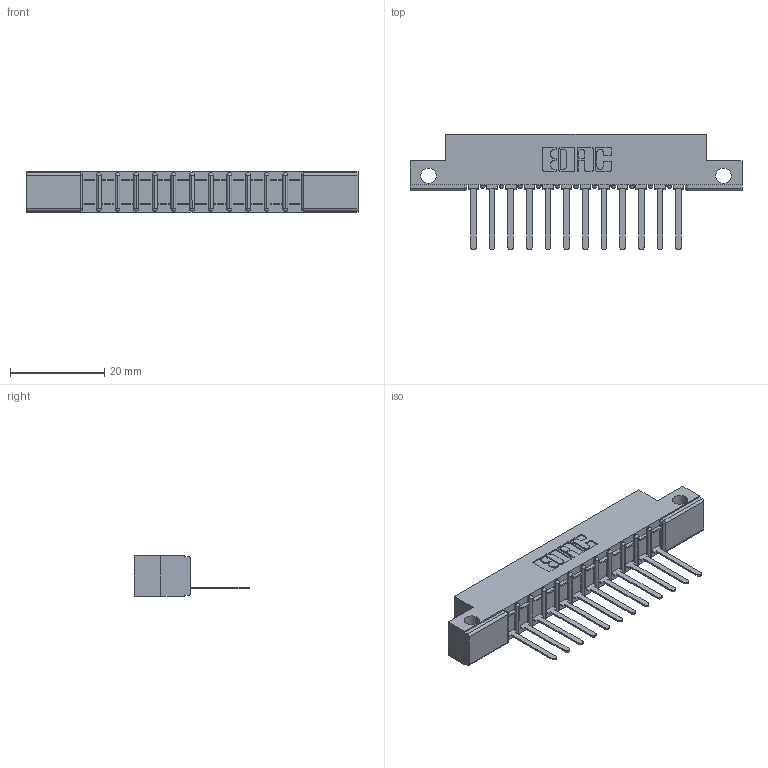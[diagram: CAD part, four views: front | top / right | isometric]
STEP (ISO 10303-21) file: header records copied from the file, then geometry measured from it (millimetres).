
FILE_DESCRIPTION (( 'STEP AP203' ), '1' );
FILE_NAME ('357-012-541-112.STEP', '2019-09-16T19:13:20', ( '' ), ( '' ), 'SwSTEP 2.0', 'SolidWorks 2016', '' );
FILE_SCHEMA (( 'CONFIG_CONTROL_DESIGN' ));
Length unit declared in the file: inch
Products named in the file (3): 307 Part_.128 Dia Side Mounting Holes; 307-290-002_541; 357-012-541-112
Assembly tree (13 placements, depth 2):
  357-012-541-112
    307 Part_.128 Dia Side Mounting Holes
    307-290-002_541  x12
Bounding box: 70.56 x 24.59 x 8.71 mm (x, y, z)
Volume: 4611 mm3; surface area: 7897.6 mm2
Topology: 13 solids, 13 shells, 1019 faces, 3107 edges, 2034 vertices
Faces by surface type: plane 610, cylinder 383, sphere 26
Entity records: 14706 total; most frequent: CARTESIAN_POINT 2476, ORIENTED_EDGE 2466, DIRECTION 2419, EDGE_CURVE 1233, LINE 929, VECTOR 929, VERTEX_POINT 802, AXIS2_PLACEMENT_3D 745
